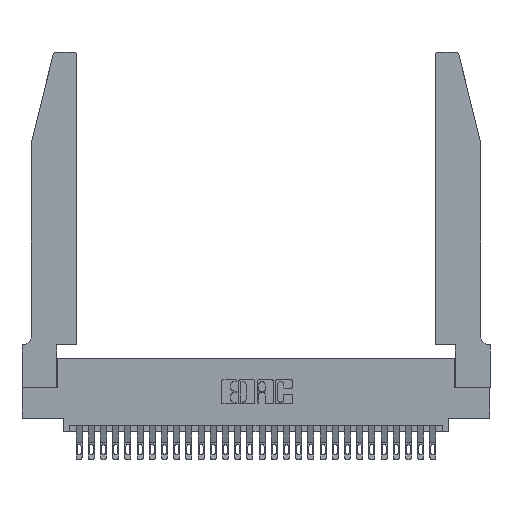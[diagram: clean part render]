
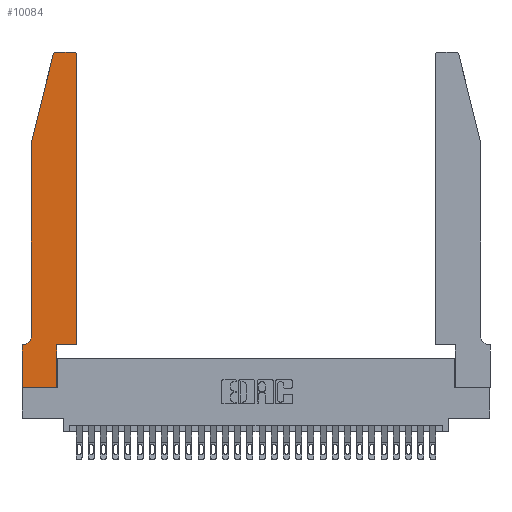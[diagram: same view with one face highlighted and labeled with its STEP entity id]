
A CAD part, top view. The second image highlights one B-rep face of the part: STEP entity #10084.
In plain terms, the highlighted planar face has unit normal (0, 0, 1).
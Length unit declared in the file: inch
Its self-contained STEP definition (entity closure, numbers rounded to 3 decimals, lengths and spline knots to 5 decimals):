
#134 = CARTESIAN_POINT ( 'NONE',  ( 0.0755, 0.35, 0.37 ) ) ;
#300 = CARTESIAN_POINT ( 'NONE',  ( 0.4205, 2.72, 0.37 ) ) ;
#920 = EDGE_CURVE ( 'NONE', #27729, #6471, #15509, .T. ) ;
#1092 = CARTESIAN_POINT ( 'NONE',  ( 0., 0., 0.37 ) ) ;
#1433 = VERTEX_POINT ( 'NONE', #26390 ) ;
#2038 = FACE_OUTER_BOUND ( 'NONE', #8621, .T. ) ;
#2128 = EDGE_CURVE ( 'NONE', #2988, #22072, #16546, .T. ) ;
#2209 = DIRECTION ( 'NONE',  ( 1., 0., 0. ) ) ;
#2422 = CARTESIAN_POINT ( 'NONE',  ( 0.284, 2.75, 0.37 ) ) ;
#2725 = DIRECTION ( 'NONE',  ( 1., 0., 0. ) ) ;
#2988 = VERTEX_POINT ( 'NONE', #11172 ) ;
#3531 = ORIENTED_EDGE ( 'NONE', *, *, #2128, .T. ) ;
#4237 = CARTESIAN_POINT ( 'NONE',  ( 0., 0., 0.37 ) ) ;
#4518 = CARTESIAN_POINT ( 'NONE',  ( 0.2605, 2.75, 0.37 ) ) ;
#4862 = CIRCLE ( 'NONE', #27224, 0.03 ) ;
#5066 = ORIENTED_EDGE ( 'NONE', *, *, #920, .T. ) ;
#5337 = EDGE_CURVE ( 'NONE', #22072, #13570, #6466, .T. ) ;
#5435 = CARTESIAN_POINT ( 'NONE',  ( 0., 0.35, 0.37 ) ) ;
#5465 = CARTESIAN_POINT ( 'NONE',  ( 0.0755, 0.42, 0.37 ) ) ;
#5959 = PLANE ( 'NONE',  #10800 ) ;
#6226 = VERTEX_POINT ( 'NONE', #21361 ) ;
#6466 = LINE ( 'NONE', #16009, #18242 ) ;
#6471 = VERTEX_POINT ( 'NONE', #24491 ) ;
#6501 = AXIS2_PLACEMENT_3D ( 'NONE', #30270, #16406, #2209 ) ;
#6743 = ORIENTED_EDGE ( 'NONE', *, *, #29023, .T. ) ;
#6995 = VECTOR ( 'NONE', #19790, 39.37008 ) ;
#7377 = DIRECTION ( 'NONE',  ( -1., 0., 0. ) ) ;
#7399 = CARTESIAN_POINT ( 'NONE',  ( 0.0755, 2., 0.37 ) ) ;
#7749 = LINE ( 'NONE', #17442, #6995 ) ;
#8488 = ORIENTED_EDGE ( 'NONE', *, *, #5337, .T. ) ;
#8621 = EDGE_LOOP ( 'NONE', ( #10388, #17955, #3531, #8488, #9464, #25759, #14839, #5066, #6743, #16788, #19781, #28112 ) ) ;
#9037 = DIRECTION ( 'NONE',  ( 0., 0., -1. ) ) ;
#9464 = ORIENTED_EDGE ( 'NONE', *, *, #12664, .T. ) ;
#9665 = EDGE_CURVE ( 'NONE', #1433, #28703, #18714, .T. ) ;
#10084 = ADVANCED_FACE ( 'NONE', ( #2038 ), #5959, .T. ) ;
#10124 = VERTEX_POINT ( 'NONE', #27128 ) ;
#10387 = VERTEX_POINT ( 'NONE', #25688 ) ;
#10388 = ORIENTED_EDGE ( 'NONE', *, *, #9665, .T. ) ;
#10702 = DIRECTION ( 'NONE',  ( 1., 0., 0. ) ) ;
#10800 = AXIS2_PLACEMENT_3D ( 'NONE', #22383, #24703, #10702 ) ;
#11172 = CARTESIAN_POINT ( 'NONE',  ( 0.25487, 2.72718, 0.37 ) ) ;
#11376 = DIRECTION ( 'NONE',  ( 0., -1., 0. ) ) ;
#11393 = LINE ( 'NONE', #27046, #29213 ) ;
#11497 = CARTESIAN_POINT ( 'NONE',  ( 0.4505, 0.35, 0.37 ) ) ;
#11548 = DIRECTION ( 'NONE',  ( -1., 0., 0. ) ) ;
#12282 = VECTOR ( 'NONE', #7377, 39.37008 ) ;
#12313 = VERTEX_POINT ( 'NONE', #5435 ) ;
#12664 = EDGE_CURVE ( 'NONE', #13570, #10124, #20077, .T. ) ;
#12713 = VERTEX_POINT ( 'NONE', #11497 ) ;
#13570 = VERTEX_POINT ( 'NONE', #5465 ) ;
#13715 = DIRECTION ( 'NONE',  ( 0., -1., 0. ) ) ;
#13842 = EDGE_CURVE ( 'NONE', #6226, #12713, #14107, .T. ) ;
#14107 = LINE ( 'NONE', #16386, #25790 ) ;
#14839 = ORIENTED_EDGE ( 'NONE', *, *, #26702, .T. ) ;
#15509 = LINE ( 'NONE', #29562, #27162 ) ;
#15826 = VECTOR ( 'NONE', #21463, 39.37008 ) ;
#16009 = CARTESIAN_POINT ( 'NONE',  ( 0.0755, 2., 0.37 ) ) ;
#16386 = CARTESIAN_POINT ( 'NONE',  ( 0.4505, 0.35, 0.37 ) ) ;
#16406 = DIRECTION ( 'NONE',  ( 0., 0., 1. ) ) ;
#16546 = LINE ( 'NONE', #7399, #15826 ) ;
#16788 = ORIENTED_EDGE ( 'NONE', *, *, #13842, .T. ) ;
#16896 = DIRECTION ( 'NONE',  ( 0., 0., 1. ) ) ;
#17022 = VECTOR ( 'NONE', #11376, 39.37008 ) ;
#17442 = CARTESIAN_POINT ( 'NONE',  ( 0.4505, 0.35, 0.37 ) ) ;
#17955 = ORIENTED_EDGE ( 'NONE', *, *, #28624, .T. ) ;
#18242 = VECTOR ( 'NONE', #13715, 39.37008 ) ;
#18546 = LINE ( 'NONE', #134, #12282 ) ;
#18714 = LINE ( 'NONE', #4518, #24897 ) ;
#18743 = DIRECTION ( 'NONE',  ( 1., 0., 0. ) ) ;
#19781 = ORIENTED_EDGE ( 'NONE', *, *, #28239, .T. ) ;
#19790 = DIRECTION ( 'NONE',  ( 0., 1., 0. ) ) ;
#20077 = CIRCLE ( 'NONE', #25511, 0.07 ) ;
#20118 = DIRECTION ( 'NONE',  ( 1., 0., 0. ) ) ;
#20173 = DIRECTION ( 'NONE',  ( 0., 1., 0. ) ) ;
#21361 = CARTESIAN_POINT ( 'NONE',  ( 0.2865, 0.35, 0.37 ) ) ;
#21463 = DIRECTION ( 'NONE',  ( -0.239, -0.971, 0. ) ) ;
#22072 = VERTEX_POINT ( 'NONE', #25624 ) ;
#22383 = CARTESIAN_POINT ( 'NONE',  ( 0., 0.35, 0.37 ) ) ;
#22402 = CIRCLE ( 'NONE', #6501, 0.03 ) ;
#23061 = CARTESIAN_POINT ( 'NONE',  ( 0.0055, 0.42, 0.37 ) ) ;
#23226 = LINE ( 'NONE', #4237, #17022 ) ;
#24491 = CARTESIAN_POINT ( 'NONE',  ( 0.2865, 0., 0.37 ) ) ;
#24703 = DIRECTION ( 'NONE',  ( 0., 0., 1. ) ) ;
#24897 = VECTOR ( 'NONE', #11548, 39.37008 ) ;
#25383 = DIRECTION ( 'NONE',  ( -1., 0., 0. ) ) ;
#25511 = AXIS2_PLACEMENT_3D ( 'NONE', #23061, #9037, #25383 ) ;
#25624 = CARTESIAN_POINT ( 'NONE',  ( 0.0755, 2., 0.37 ) ) ;
#25688 = CARTESIAN_POINT ( 'NONE',  ( 0.4505, 2.72, 0.37 ) ) ;
#25759 = ORIENTED_EDGE ( 'NONE', *, *, #26212, .T. ) ;
#25790 = VECTOR ( 'NONE', #18743, 39.37008 ) ;
#26212 = EDGE_CURVE ( 'NONE', #10124, #12313, #18546, .T. ) ;
#26390 = CARTESIAN_POINT ( 'NONE',  ( 0.4205, 2.75, 0.37 ) ) ;
#26702 = EDGE_CURVE ( 'NONE', #12313, #27729, #23226, .T. ) ;
#26965 = EDGE_CURVE ( 'NONE', #10387, #1433, #4862, .T. ) ;
#27046 = CARTESIAN_POINT ( 'NONE',  ( 0.2865, 0.35, 0.37 ) ) ;
#27128 = CARTESIAN_POINT ( 'NONE',  ( 0.0055, 0.35, 0.37 ) ) ;
#27162 = VECTOR ( 'NONE', #20118, 39.37008 ) ;
#27224 = AXIS2_PLACEMENT_3D ( 'NONE', #300, #16896, #2725 ) ;
#27729 = VERTEX_POINT ( 'NONE', #1092 ) ;
#28112 = ORIENTED_EDGE ( 'NONE', *, *, #26965, .T. ) ;
#28239 = EDGE_CURVE ( 'NONE', #12713, #10387, #7749, .T. ) ;
#28624 = EDGE_CURVE ( 'NONE', #28703, #2988, #22402, .T. ) ;
#28703 = VERTEX_POINT ( 'NONE', #2422 ) ;
#29023 = EDGE_CURVE ( 'NONE', #6471, #6226, #11393, .T. ) ;
#29213 = VECTOR ( 'NONE', #20173, 39.37008 ) ;
#29562 = CARTESIAN_POINT ( 'NONE',  ( 0., 0., 0.37 ) ) ;
#30270 = CARTESIAN_POINT ( 'NONE',  ( 0.284, 2.72, 0.37 ) ) ;
